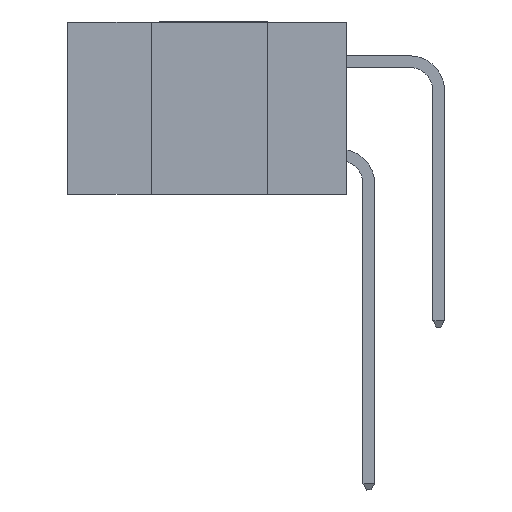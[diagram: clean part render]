
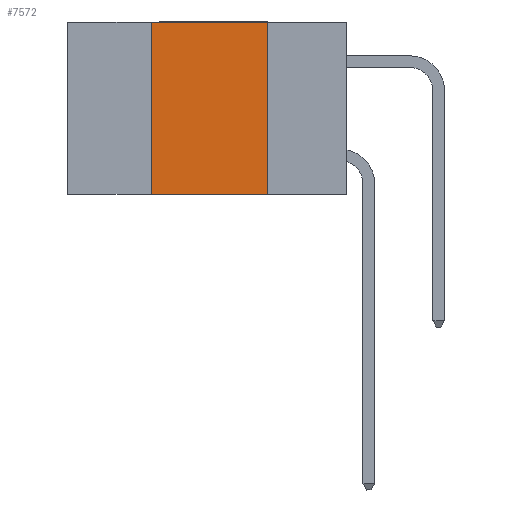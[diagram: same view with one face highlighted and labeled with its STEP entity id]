
A CAD part, left-side view. The second image highlights one B-rep face of the part: STEP entity #7572.
In plain terms, the highlighted planar face has unit normal (-1, 0, 0).
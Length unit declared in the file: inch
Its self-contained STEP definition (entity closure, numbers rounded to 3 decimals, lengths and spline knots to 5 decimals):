
#113 = CARTESIAN_POINT ( 'NONE',  ( 0., 0.42, 0. ) ) ;
#130 = ORIENTED_EDGE ( 'NONE', *, *, #9254, .F. ) ;
#317 = VERTEX_POINT ( 'NONE', #8349 ) ;
#463 = VERTEX_POINT ( 'NONE', #6178 ) ;
#582 = LINE ( 'NONE', #6334, #10104 ) ;
#1669 = DIRECTION ( 'NONE',  ( 0., 0., -1. ) ) ;
#1962 = EDGE_CURVE ( 'NONE', #317, #5776, #8333, .T. ) ;
#3109 = VECTOR ( 'NONE', #10558, 39.37008 ) ;
#3177 = VECTOR ( 'NONE', #5877, 39.37008 ) ;
#3311 = CARTESIAN_POINT ( 'NONE',  ( 0., 0.42, 0. ) ) ;
#3458 = ORIENTED_EDGE ( 'NONE', *, *, #5770, .T. ) ;
#3514 = DIRECTION ( 'NONE',  ( 0., -1., 0. ) ) ;
#3552 = PLANE ( 'NONE',  #10654 ) ;
#3724 = CARTESIAN_POINT ( 'NONE',  ( 0., 0.17, 0. ) ) ;
#3795 = LINE ( 'NONE', #3892, #5741 ) ;
#3892 = CARTESIAN_POINT ( 'NONE',  ( 0., 0.17, 0. ) ) ;
#4453 = VERTEX_POINT ( 'NONE', #3724 ) ;
#4583 = EDGE_CURVE ( 'NONE', #4453, #463, #3795, .T. ) ;
#5735 = LINE ( 'NONE', #9394, #3177 ) ;
#5741 = VECTOR ( 'NONE', #6729, 39.37008 ) ;
#5770 = EDGE_CURVE ( 'NONE', #317, #463, #5735, .T. ) ;
#5776 = VERTEX_POINT ( 'NONE', #113 ) ;
#5877 = DIRECTION ( 'NONE',  ( 0., -1., 0. ) ) ;
#6178 = CARTESIAN_POINT ( 'NONE',  ( 0., 0.17, -0.37 ) ) ;
#6263 = ORIENTED_EDGE ( 'NONE', *, *, #4583, .F. ) ;
#6334 = CARTESIAN_POINT ( 'NONE',  ( 0., 0.6, 0. ) ) ;
#6729 = DIRECTION ( 'NONE',  ( 0., 0., -1. ) ) ;
#7312 = DIRECTION ( 'NONE',  ( 1., 0., 0. ) ) ;
#7572 = ADVANCED_FACE ( 'NONE', ( #7811 ), #3552, .F. ) ;
#7811 = FACE_OUTER_BOUND ( 'NONE', #8328, .T. ) ;
#8232 = ORIENTED_EDGE ( 'NONE', *, *, #1962, .F. ) ;
#8328 = EDGE_LOOP ( 'NONE', ( #6263, #130, #8232, #3458 ) ) ;
#8333 = LINE ( 'NONE', #3311, #3109 ) ;
#8349 = CARTESIAN_POINT ( 'NONE',  ( 0., 0.42, -0.37 ) ) ;
#9254 = EDGE_CURVE ( 'NONE', #5776, #4453, #582, .T. ) ;
#9394 = CARTESIAN_POINT ( 'NONE',  ( 0., 0.6, -0.37 ) ) ;
#9903 = CARTESIAN_POINT ( 'NONE',  ( 0., 0.6, 0. ) ) ;
#10104 = VECTOR ( 'NONE', #3514, 39.37008 ) ;
#10558 = DIRECTION ( 'NONE',  ( 0., 0., 1. ) ) ;
#10654 = AXIS2_PLACEMENT_3D ( 'NONE', #9903, #7312, #1669 ) ;
